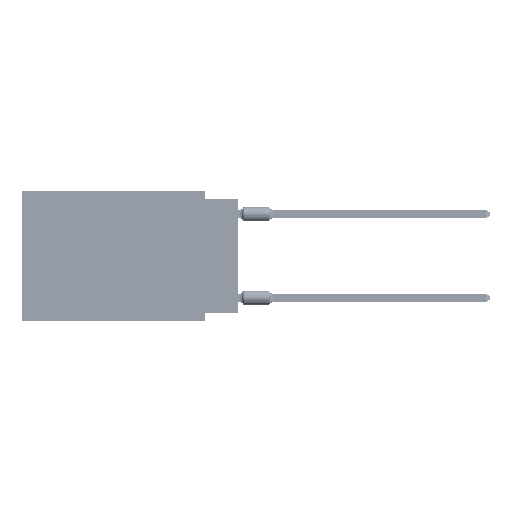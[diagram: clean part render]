
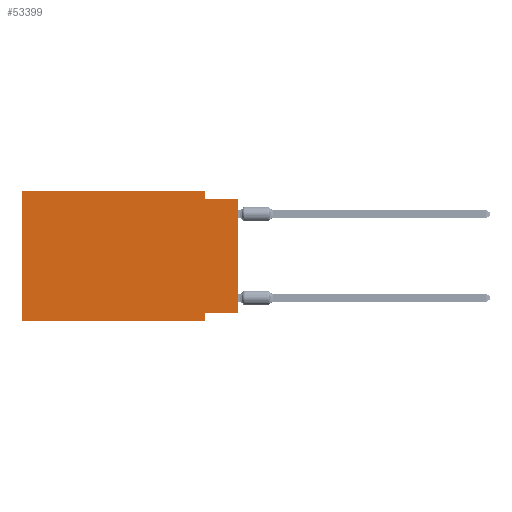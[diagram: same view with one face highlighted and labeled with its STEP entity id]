
A CAD part, left-side view. The second image highlights one B-rep face of the part: STEP entity #53399.
In plain terms, the highlighted planar face has unit normal (-1, 0, 0).
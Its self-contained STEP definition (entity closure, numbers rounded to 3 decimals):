
#350 = CARTESIAN_POINT ( 'NONE',  ( 0., 16.383, 0. ) ) ;
#470 = LINE ( 'NONE', #44296, #15689 ) ;
#2291 = ORIENTED_EDGE ( 'NONE', *, *, #57182, .F. ) ;
#3313 = DIRECTION ( 'NONE',  ( 0., 0., -1. ) ) ;
#3469 = EDGE_CURVE ( 'NONE', #39396, #31527, #65896, .T. ) ;
#5986 = CARTESIAN_POINT ( 'NONE',  ( 0., 0., -9.271 ) ) ;
#6326 = VERTEX_POINT ( 'NONE', #5986 ) ;
#7026 = VECTOR ( 'NONE', #58002, 1000. ) ;
#7462 = VECTOR ( 'NONE', #66209, 1000. ) ;
#8163 = EDGE_CURVE ( 'NONE', #25637, #59931, #21454, .T. ) ;
#9409 = ORIENTED_EDGE ( 'NONE', *, *, #34817, .F. ) ;
#11392 = EDGE_CURVE ( 'NONE', #22098, #39396, #13136, .T. ) ;
#12496 = DIRECTION ( 'NONE',  ( 0., 0., -1. ) ) ;
#12848 = CARTESIAN_POINT ( 'NONE',  ( 0., 2.54, -9.906 ) ) ;
#13136 = LINE ( 'NONE', #53347, #23687 ) ;
#15423 = CARTESIAN_POINT ( 'NONE',  ( 0., 16.383, 0. ) ) ;
#15689 = VECTOR ( 'NONE', #32164, 1000. ) ;
#17762 = CARTESIAN_POINT ( 'NONE',  ( 0., 2.54, -0.635 ) ) ;
#17949 = ORIENTED_EDGE ( 'NONE', *, *, #8163, .F. ) ;
#20414 = FACE_OUTER_BOUND ( 'NONE', #65466, .T. ) ;
#20986 = CARTESIAN_POINT ( 'NONE',  ( 0., 16.383, -9.906 ) ) ;
#21154 = EDGE_CURVE ( 'NONE', #6326, #59931, #44837, .T. ) ;
#21454 = LINE ( 'NONE', #69206, #50743 ) ;
#21988 = VERTEX_POINT ( 'NONE', #12848 ) ;
#22020 = VECTOR ( 'NONE', #49151, 1000. ) ;
#22098 = VERTEX_POINT ( 'NONE', #20986 ) ;
#22571 = VECTOR ( 'NONE', #12496, 1000. ) ;
#23687 = VECTOR ( 'NONE', #64743, 1000. ) ;
#25224 = CARTESIAN_POINT ( 'NONE',  ( 0., 0., -9.271 ) ) ;
#25637 = VERTEX_POINT ( 'NONE', #17762 ) ;
#27351 = EDGE_CURVE ( 'NONE', #31527, #25637, #52837, .T. ) ;
#28789 = EDGE_CURVE ( 'NONE', #22098, #21988, #470, .T. ) ;
#31527 = VERTEX_POINT ( 'NONE', #42494 ) ;
#32158 = PLANE ( 'NONE',  #33783 ) ;
#32164 = DIRECTION ( 'NONE',  ( 0., -1., 0. ) ) ;
#32783 = ORIENTED_EDGE ( 'NONE', *, *, #28789, .T. ) ;
#33783 = AXIS2_PLACEMENT_3D ( 'NONE', #15423, #42149, #64940 ) ;
#34817 = EDGE_CURVE ( 'NONE', #6326, #50406, #48013, .T. ) ;
#34925 = LINE ( 'NONE', #66997, #22571 ) ;
#35448 = ORIENTED_EDGE ( 'NONE', *, *, #3469, .F. ) ;
#36085 = ORIENTED_EDGE ( 'NONE', *, *, #11392, .F. ) ;
#39396 = VERTEX_POINT ( 'NONE', #46483 ) ;
#40949 = CARTESIAN_POINT ( 'NONE',  ( 0., 0., -0.635 ) ) ;
#42149 = DIRECTION ( 'NONE',  ( 1., 0., 0. ) ) ;
#42494 = CARTESIAN_POINT ( 'NONE',  ( 0., 2.54, 0. ) ) ;
#44296 = CARTESIAN_POINT ( 'NONE',  ( 0., 16.383, -9.906 ) ) ;
#44837 = LINE ( 'NONE', #67257, #7462 ) ;
#46483 = CARTESIAN_POINT ( 'NONE',  ( 0., 16.383, 0. ) ) ;
#48013 = LINE ( 'NONE', #25224, #7026 ) ;
#49151 = DIRECTION ( 'NONE',  ( 0., -1., 0. ) ) ;
#50406 = VERTEX_POINT ( 'NONE', #60216 ) ;
#50743 = VECTOR ( 'NONE', #63855, 1000. ) ;
#52837 = LINE ( 'NONE', #62828, #56387 ) ;
#53347 = CARTESIAN_POINT ( 'NONE',  ( 0., 16.383, 0. ) ) ;
#53399 = ADVANCED_FACE ( 'NONE', ( #20414 ), #32158, .F. ) ;
#55357 = ORIENTED_EDGE ( 'NONE', *, *, #21154, .T. ) ;
#56387 = VECTOR ( 'NONE', #3313, 1000. ) ;
#57182 = EDGE_CURVE ( 'NONE', #50406, #21988, #34925, .T. ) ;
#58002 = DIRECTION ( 'NONE',  ( 0., 1., 0. ) ) ;
#59931 = VERTEX_POINT ( 'NONE', #40949 ) ;
#60216 = CARTESIAN_POINT ( 'NONE',  ( 0., 2.54, -9.271 ) ) ;
#62828 = CARTESIAN_POINT ( 'NONE',  ( 0., 2.54, 0. ) ) ;
#63855 = DIRECTION ( 'NONE',  ( 0., -1., 0. ) ) ;
#64743 = DIRECTION ( 'NONE',  ( 0., 0., 1. ) ) ;
#64940 = DIRECTION ( 'NONE',  ( 0., 0., -1. ) ) ;
#65466 = EDGE_LOOP ( 'NONE', ( #55357, #17949, #68310, #35448, #36085, #32783, #2291, #9409 ) ) ;
#65896 = LINE ( 'NONE', #350, #22020 ) ;
#66209 = DIRECTION ( 'NONE',  ( 0., 0., 1. ) ) ;
#66997 = CARTESIAN_POINT ( 'NONE',  ( 0., 2.54, -9.906 ) ) ;
#67257 = CARTESIAN_POINT ( 'NONE',  ( 0., 0., 0. ) ) ;
#68310 = ORIENTED_EDGE ( 'NONE', *, *, #27351, .F. ) ;
#69206 = CARTESIAN_POINT ( 'NONE',  ( 0., 0., -0.635 ) ) ;
